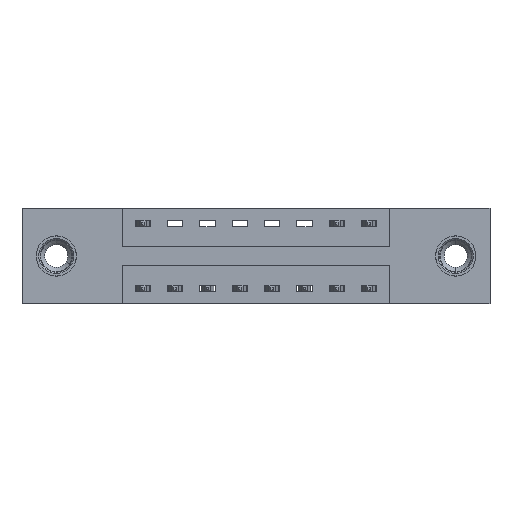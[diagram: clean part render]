
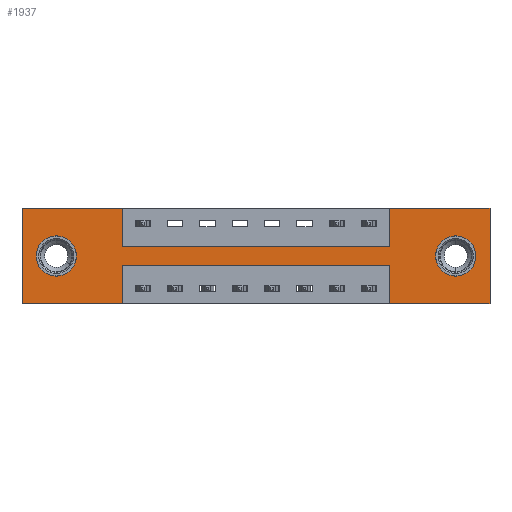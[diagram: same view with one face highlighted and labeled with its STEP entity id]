
A CAD part, front view. The second image highlights one B-rep face of the part: STEP entity #1937.
In plain terms, the highlighted planar face has unit normal (0, -1, 0).
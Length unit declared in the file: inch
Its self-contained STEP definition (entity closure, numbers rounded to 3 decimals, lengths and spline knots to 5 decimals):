
#15 = ORIENTED_EDGE ( 'NONE', *, *, #10792, .F. ) ;
#101 = ORIENTED_EDGE ( 'NONE', *, *, #9818, .T. ) ;
#111 = VERTEX_POINT ( 'NONE', #9278 ) ;
#142 = CIRCLE ( 'NONE', #2102, 0.078 ) ;
#196 = CIRCLE ( 'NONE', #3077, 0.078 ) ;
#315 = ORIENTED_EDGE ( 'NONE', *, *, #4894, .T. ) ;
#430 = VERTEX_POINT ( 'NONE', #2471 ) ;
#519 = EDGE_CURVE ( 'NONE', #2344, #2103, #3222, .T. ) ;
#550 = CARTESIAN_POINT ( 'NONE',  ( 1.6775, 0., -0.263 ) ) ;
#572 = VECTOR ( 'NONE', #7663, 39.37008 ) ;
#626 = CIRCLE ( 'NONE', #2509, 0.078 ) ;
#719 = ORIENTED_EDGE ( 'NONE', *, *, #3531, .F. ) ;
#882 = DIRECTION ( 'NONE',  ( -1., 0., 0. ) ) ;
#894 = LINE ( 'NONE', #4116, #9063 ) ;
#898 = VECTOR ( 'NONE', #4301, 39.37008 ) ;
#1019 = VERTEX_POINT ( 'NONE', #5167 ) ;
#1187 = DIRECTION ( 'NONE',  ( 0., -1., 0. ) ) ;
#1251 = VERTEX_POINT ( 'NONE', #7136 ) ;
#1270 = CARTESIAN_POINT ( 'NONE',  ( 1.4225, 0., -0.15 ) ) ;
#1316 = VERTEX_POINT ( 'NONE', #7270 ) ;
#1404 = DIRECTION ( 'NONE',  ( 0., 0., 1. ) ) ;
#1472 = DIRECTION ( 'NONE',  ( 0., 0., 1. ) ) ;
#1495 = DIRECTION ( 'NONE',  ( -1., 0., 0. ) ) ;
#1523 = AXIS2_PLACEMENT_3D ( 'NONE', #5566, #1187, #7223 ) ;
#1698 = LINE ( 'NONE', #3404, #6040 ) ;
#1816 = VERTEX_POINT ( 'NONE', #9396 ) ;
#1819 = VERTEX_POINT ( 'NONE', #2788 ) ;
#1937 = ADVANCED_FACE ( 'NONE', ( #2369, #10597, #2095 ), #6407, .T. ) ;
#2095 = FACE_OUTER_BOUND ( 'NONE', #3517, .T. ) ;
#2102 = AXIS2_PLACEMENT_3D ( 'NONE', #9540, #4760, #10339 ) ;
#2103 = VERTEX_POINT ( 'NONE', #550 ) ;
#2115 = EDGE_CURVE ( 'NONE', #111, #1019, #2490, .T. ) ;
#2272 = CARTESIAN_POINT ( 'NONE',  ( 0.1325, 0., -0.107 ) ) ;
#2339 = LINE ( 'NONE', #7942, #10327 ) ;
#2344 = VERTEX_POINT ( 'NONE', #7736 ) ;
#2348 = DIRECTION ( 'NONE',  ( 0., 1., 0. ) ) ;
#2369 = FACE_BOUND ( 'NONE', #7746, .T. ) ;
#2471 = CARTESIAN_POINT ( 'NONE',  ( 0.3875, 0., -0.15 ) ) ;
#2490 = LINE ( 'NONE', #6649, #7045 ) ;
#2509 = AXIS2_PLACEMENT_3D ( 'NONE', #7441, #2348, #8249 ) ;
#2524 = LINE ( 'NONE', #6937, #2800 ) ;
#2614 = CARTESIAN_POINT ( 'NONE',  ( 0.3875, 0., 0. ) ) ;
#2788 = CARTESIAN_POINT ( 'NONE',  ( 0.3875, 0., 0. ) ) ;
#2800 = VECTOR ( 'NONE', #882, 39.37008 ) ;
#2825 = ORIENTED_EDGE ( 'NONE', *, *, #4932, .F. ) ;
#3001 = LINE ( 'NONE', #4673, #7502 ) ;
#3077 = AXIS2_PLACEMENT_3D ( 'NONE', #9965, #5201, #10746 ) ;
#3222 = CIRCLE ( 'NONE', #9657, 0.078 ) ;
#3299 = VERTEX_POINT ( 'NONE', #9440 ) ;
#3322 = EDGE_CURVE ( 'NONE', #5045, #3299, #2339, .T. ) ;
#3377 = CARTESIAN_POINT ( 'NONE',  ( 0.3875, 0., -0.15 ) ) ;
#3404 = CARTESIAN_POINT ( 'NONE',  ( 0.3875, 0., -0.37 ) ) ;
#3474 = CARTESIAN_POINT ( 'NONE',  ( 1.81, 0., 0. ) ) ;
#3517 = EDGE_LOOP ( 'NONE', ( #15, #8462, #5180, #8674, #6409, #6578, #8701, #4915, #2825, #5175, #9412, #719 ) ) ;
#3531 = EDGE_CURVE ( 'NONE', #10161, #111, #10442, .T. ) ;
#3539 = CARTESIAN_POINT ( 'NONE',  ( 1.6775, 0., -0.185 ) ) ;
#3591 = CARTESIAN_POINT ( 'NONE',  ( 0., 0., 0. ) ) ;
#3839 = LINE ( 'NONE', #7187, #7991 ) ;
#4116 = CARTESIAN_POINT ( 'NONE',  ( 1.4225, 0., -0.37 ) ) ;
#4267 = CARTESIAN_POINT ( 'NONE',  ( 0.3875, 0., -0.37 ) ) ;
#4301 = DIRECTION ( 'NONE',  ( 1., 0., 0. ) ) ;
#4413 = LINE ( 'NONE', #2614, #6877 ) ;
#4447 = DIRECTION ( 'NONE',  ( 0., 0., -1. ) ) ;
#4571 = CARTESIAN_POINT ( 'NONE',  ( 1.4225, 0., 0. ) ) ;
#4673 = CARTESIAN_POINT ( 'NONE',  ( 1.4225, 0., 0. ) ) ;
#4760 = DIRECTION ( 'NONE',  ( 0., 1., 0. ) ) ;
#4894 = EDGE_CURVE ( 'NONE', #6085, #9296, #196, .T. ) ;
#4915 = ORIENTED_EDGE ( 'NONE', *, *, #5477, .F. ) ;
#4932 = EDGE_CURVE ( 'NONE', #1819, #430, #4413, .T. ) ;
#5045 = VERTEX_POINT ( 'NONE', #4571 ) ;
#5092 = EDGE_LOOP ( 'NONE', ( #101, #315 ) ) ;
#5167 = CARTESIAN_POINT ( 'NONE',  ( 0., 0., 0. ) ) ;
#5175 = ORIENTED_EDGE ( 'NONE', *, *, #5648, .F. ) ;
#5180 = ORIENTED_EDGE ( 'NONE', *, *, #8712, .F. ) ;
#5201 = DIRECTION ( 'NONE',  ( 0., 1., 0. ) ) ;
#5477 = EDGE_CURVE ( 'NONE', #430, #7281, #9547, .T. ) ;
#5502 = DIRECTION ( 'NONE',  ( 0., 0., 1. ) ) ;
#5566 = CARTESIAN_POINT ( 'NONE',  ( 0., 0., -0.37 ) ) ;
#5648 = EDGE_CURVE ( 'NONE', #1019, #1819, #6221, .T. ) ;
#5740 = CARTESIAN_POINT ( 'NONE',  ( 0.1325, 0., -0.263 ) ) ;
#5829 = EDGE_CURVE ( 'NONE', #9868, #1316, #3839, .T. ) ;
#6040 = VECTOR ( 'NONE', #6785, 39.37008 ) ;
#6085 = VERTEX_POINT ( 'NONE', #5740 ) ;
#6221 = LINE ( 'NONE', #3591, #8117 ) ;
#6407 = PLANE ( 'NONE',  #1523 ) ;
#6409 = ORIENTED_EDGE ( 'NONE', *, *, #9542, .F. ) ;
#6578 = ORIENTED_EDGE ( 'NONE', *, *, #3322, .F. ) ;
#6649 = CARTESIAN_POINT ( 'NONE',  ( 0., 0., 0. ) ) ;
#6686 = EDGE_CURVE ( 'NONE', #2103, #2344, #626, .T. ) ;
#6785 = DIRECTION ( 'NONE',  ( 0., 0., -1. ) ) ;
#6877 = VECTOR ( 'NONE', #8482, 39.37008 ) ;
#6937 = CARTESIAN_POINT ( 'NONE',  ( 0.3875, 0., -0.22 ) ) ;
#7045 = VECTOR ( 'NONE', #1472, 39.37008 ) ;
#7135 = EDGE_CURVE ( 'NONE', #7281, #5045, #3001, .T. ) ;
#7136 = CARTESIAN_POINT ( 'NONE',  ( 0.3875, 0., -0.22 ) ) ;
#7187 = CARTESIAN_POINT ( 'NONE',  ( 0., 0., -0.37 ) ) ;
#7223 = DIRECTION ( 'NONE',  ( 0., 0., -1. ) ) ;
#7270 = CARTESIAN_POINT ( 'NONE',  ( 1.4225, 0., -0.37 ) ) ;
#7281 = VERTEX_POINT ( 'NONE', #1270 ) ;
#7441 = CARTESIAN_POINT ( 'NONE',  ( 1.6775, 0., -0.185 ) ) ;
#7502 = VECTOR ( 'NONE', #5502, 39.37008 ) ;
#7663 = DIRECTION ( 'NONE',  ( 0., 0., -1. ) ) ;
#7736 = CARTESIAN_POINT ( 'NONE',  ( 1.6775, 0., -0.107 ) ) ;
#7746 = EDGE_LOOP ( 'NONE', ( #10513, #8431 ) ) ;
#7942 = CARTESIAN_POINT ( 'NONE',  ( 0., 0., 0. ) ) ;
#7991 = VECTOR ( 'NONE', #8766, 39.37008 ) ;
#8117 = VECTOR ( 'NONE', #8871, 39.37008 ) ;
#8249 = DIRECTION ( 'NONE',  ( 0., 0., -1. ) ) ;
#8386 = VECTOR ( 'NONE', #1495, 39.37008 ) ;
#8431 = ORIENTED_EDGE ( 'NONE', *, *, #6686, .T. ) ;
#8462 = ORIENTED_EDGE ( 'NONE', *, *, #10269, .F. ) ;
#8482 = DIRECTION ( 'NONE',  ( 0., 0., -1. ) ) ;
#8674 = ORIENTED_EDGE ( 'NONE', *, *, #5829, .F. ) ;
#8701 = ORIENTED_EDGE ( 'NONE', *, *, #7135, .F. ) ;
#8708 = DIRECTION ( 'NONE',  ( 1., 0., 0. ) ) ;
#8712 = EDGE_CURVE ( 'NONE', #1316, #1816, #894, .T. ) ;
#8766 = DIRECTION ( 'NONE',  ( -1., 0., 0. ) ) ;
#8836 = CARTESIAN_POINT ( 'NONE',  ( 1.81, 0., -0.37 ) ) ;
#8871 = DIRECTION ( 'NONE',  ( 1., 0., 0. ) ) ;
#9063 = VECTOR ( 'NONE', #1404, 39.37008 ) ;
#9251 = DIRECTION ( 'NONE',  ( 0., 1., 0. ) ) ;
#9278 = CARTESIAN_POINT ( 'NONE',  ( 0., 0., -0.37 ) ) ;
#9282 = LINE ( 'NONE', #3474, #572 ) ;
#9296 = VERTEX_POINT ( 'NONE', #2272 ) ;
#9396 = CARTESIAN_POINT ( 'NONE',  ( 1.4225, 0., -0.22 ) ) ;
#9412 = ORIENTED_EDGE ( 'NONE', *, *, #2115, .F. ) ;
#9440 = CARTESIAN_POINT ( 'NONE',  ( 1.81, 0., 0. ) ) ;
#9540 = CARTESIAN_POINT ( 'NONE',  ( 0.1325, 0., -0.185 ) ) ;
#9542 = EDGE_CURVE ( 'NONE', #3299, #9868, #9282, .T. ) ;
#9547 = LINE ( 'NONE', #3377, #898 ) ;
#9657 = AXIS2_PLACEMENT_3D ( 'NONE', #3539, #9251, #4447 ) ;
#9818 = EDGE_CURVE ( 'NONE', #9296, #6085, #142, .T. ) ;
#9868 = VERTEX_POINT ( 'NONE', #8836 ) ;
#9965 = CARTESIAN_POINT ( 'NONE',  ( 0.1325, 0., -0.185 ) ) ;
#10161 = VERTEX_POINT ( 'NONE', #4267 ) ;
#10269 = EDGE_CURVE ( 'NONE', #1816, #1251, #2524, .T. ) ;
#10327 = VECTOR ( 'NONE', #8708, 39.37008 ) ;
#10339 = DIRECTION ( 'NONE',  ( 0., 0., 1. ) ) ;
#10442 = LINE ( 'NONE', #10573, #8386 ) ;
#10513 = ORIENTED_EDGE ( 'NONE', *, *, #519, .T. ) ;
#10573 = CARTESIAN_POINT ( 'NONE',  ( 0., 0., -0.37 ) ) ;
#10597 = FACE_BOUND ( 'NONE', #5092, .T. ) ;
#10746 = DIRECTION ( 'NONE',  ( 0., 0., 1. ) ) ;
#10792 = EDGE_CURVE ( 'NONE', #1251, #10161, #1698, .T. ) ;
